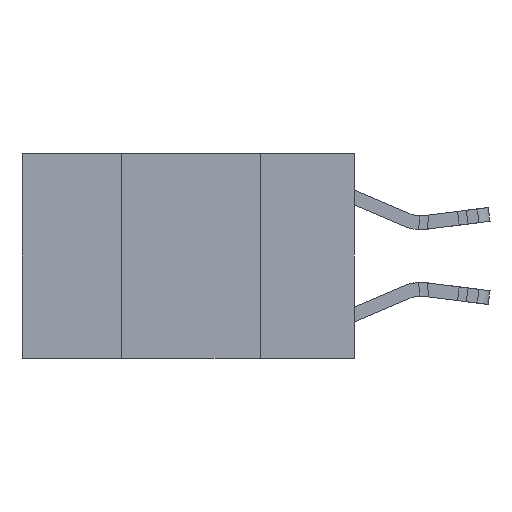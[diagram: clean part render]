
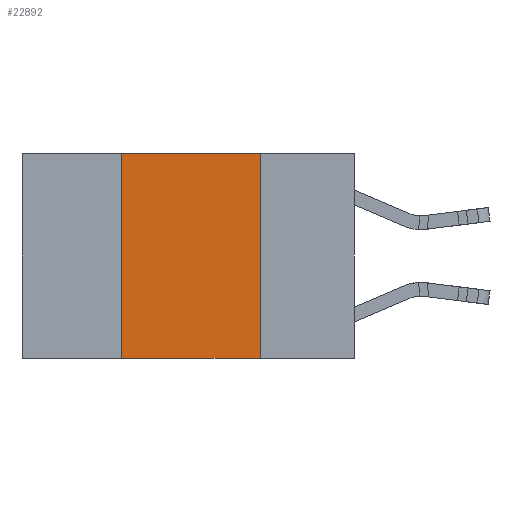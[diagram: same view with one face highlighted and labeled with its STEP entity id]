
A CAD part, left-side view. The second image highlights one B-rep face of the part: STEP entity #22892.
In plain terms, the highlighted planar face has unit normal (-1, 0, 0).
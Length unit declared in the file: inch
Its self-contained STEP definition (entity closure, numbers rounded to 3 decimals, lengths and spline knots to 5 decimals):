
#258 = CARTESIAN_POINT ( 'NONE',  ( 0., 0.17, 0. ) ) ;
#1255 = AXIS2_PLACEMENT_3D ( 'NONE', #9728, #17171, #12174 ) ;
#1358 = DIRECTION ( 'NONE',  ( 0., 0., 1. ) ) ;
#1382 = VECTOR ( 'NONE', #1358, 39.37008 ) ;
#1973 = ORIENTED_EDGE ( 'NONE', *, *, #11343, .F. ) ;
#2308 = VERTEX_POINT ( 'NONE', #30847 ) ;
#3544 = ORIENTED_EDGE ( 'NONE', *, *, #16801, .F. ) ;
#6069 = LINE ( 'NONE', #13677, #1382 ) ;
#9492 = DIRECTION ( 'NONE',  ( 0., -1., 0. ) ) ;
#9728 = CARTESIAN_POINT ( 'NONE',  ( 0., 0.6, 0. ) ) ;
#11343 = EDGE_CURVE ( 'NONE', #29078, #31325, #17643, .T. ) ;
#12174 = DIRECTION ( 'NONE',  ( 0., 0., -1. ) ) ;
#13677 = CARTESIAN_POINT ( 'NONE',  ( 0., 0.42, 0. ) ) ;
#14479 = VECTOR ( 'NONE', #20229, 39.37008 ) ;
#15838 = VECTOR ( 'NONE', #23187, 39.37008 ) ;
#16801 = EDGE_CURVE ( 'NONE', #29653, #29078, #16908, .T. ) ;
#16908 = LINE ( 'NONE', #31152, #21042 ) ;
#17171 = DIRECTION ( 'NONE',  ( 1., 0., 0. ) ) ;
#17449 = ORIENTED_EDGE ( 'NONE', *, *, #23537, .T. ) ;
#17643 = LINE ( 'NONE', #27501, #14479 ) ;
#17996 = CARTESIAN_POINT ( 'NONE',  ( 0., 0.17, -0.37 ) ) ;
#19919 = PLANE ( 'NONE',  #1255 ) ;
#20229 = DIRECTION ( 'NONE',  ( 0., 0., -1. ) ) ;
#21042 = VECTOR ( 'NONE', #9492, 39.37008 ) ;
#22892 = ADVANCED_FACE ( 'NONE', ( #24440 ), #19919, .F. ) ;
#23187 = DIRECTION ( 'NONE',  ( 0., -1., 0. ) ) ;
#23537 = EDGE_CURVE ( 'NONE', #2308, #31325, #25465, .T. ) ;
#23568 = EDGE_CURVE ( 'NONE', #2308, #29653, #6069, .T. ) ;
#24440 = FACE_OUTER_BOUND ( 'NONE', #24544, .T. ) ;
#24544 = EDGE_LOOP ( 'NONE', ( #1973, #3544, #25248, #17449 ) ) ;
#25248 = ORIENTED_EDGE ( 'NONE', *, *, #23568, .F. ) ;
#25465 = LINE ( 'NONE', #25934, #15838 ) ;
#25934 = CARTESIAN_POINT ( 'NONE',  ( 0., 0.6, -0.37 ) ) ;
#27501 = CARTESIAN_POINT ( 'NONE',  ( 0., 0.17, 0. ) ) ;
#29078 = VERTEX_POINT ( 'NONE', #258 ) ;
#29653 = VERTEX_POINT ( 'NONE', #31019 ) ;
#30847 = CARTESIAN_POINT ( 'NONE',  ( 0., 0.42, -0.37 ) ) ;
#31019 = CARTESIAN_POINT ( 'NONE',  ( 0., 0.42, 0. ) ) ;
#31152 = CARTESIAN_POINT ( 'NONE',  ( 0., 0.6, 0. ) ) ;
#31325 = VERTEX_POINT ( 'NONE', #17996 ) ;
